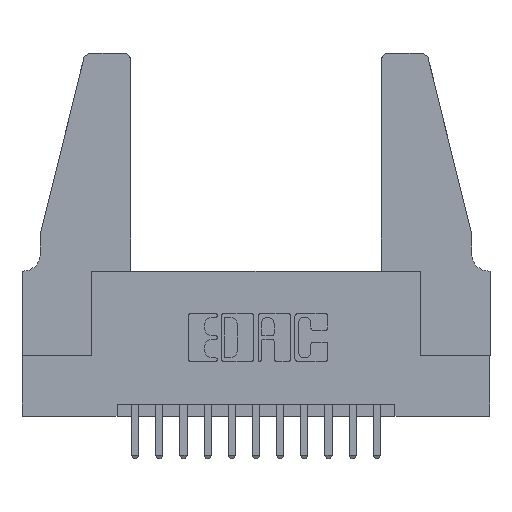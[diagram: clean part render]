
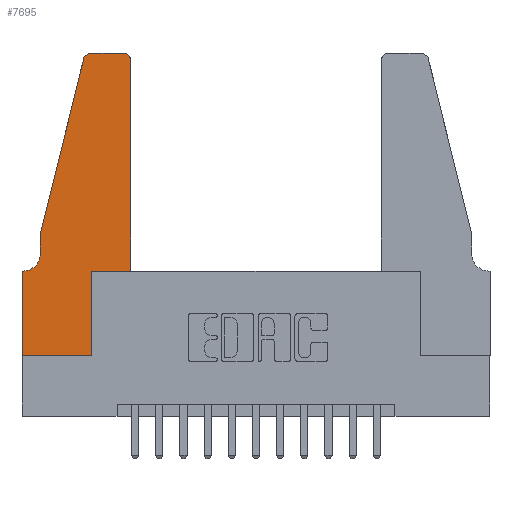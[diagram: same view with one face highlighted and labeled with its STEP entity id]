
A CAD part, top view. The second image highlights one B-rep face of the part: STEP entity #7695.
In plain terms, the highlighted planar face has unit normal (0, 0, 1).
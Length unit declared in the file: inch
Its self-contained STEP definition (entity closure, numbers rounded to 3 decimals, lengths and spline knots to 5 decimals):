
#116 = LINE ( 'NONE', #12809, #12849 ) ;
#664 = CARTESIAN_POINT ( 'NONE',  ( 0., 0., 0.37 ) ) ;
#724 = DIRECTION ( 'NONE',  ( 1., 0., 0. ) ) ;
#802 = ORIENTED_EDGE ( 'NONE', *, *, #12602, .T. ) ;
#809 = DIRECTION ( 'NONE',  ( -1., 0., 0. ) ) ;
#882 = ORIENTED_EDGE ( 'NONE', *, *, #12974, .T. ) ;
#1076 = VECTOR ( 'NONE', #12308, 39.37008 ) ;
#1190 = CARTESIAN_POINT ( 'NONE',  ( 0.0755, 0.5, 0.37 ) ) ;
#1233 = LINE ( 'NONE', #2793, #14843 ) ;
#1574 = VERTEX_POINT ( 'NONE', #13726 ) ;
#1674 = DIRECTION ( 'NONE',  ( 0., 1., 0. ) ) ;
#1694 = CARTESIAN_POINT ( 'NONE',  ( 0.284, 1.22, 0.37 ) ) ;
#1744 = VECTOR ( 'NONE', #14586, 39.37008 ) ;
#1784 = DIRECTION ( 'NONE',  ( 0., 0., 1. ) ) ;
#1960 = CIRCLE ( 'NONE', #13299, 0.03 ) ;
#2003 = CARTESIAN_POINT ( 'NONE',  ( 0.0055, 0.42, 0.37 ) ) ;
#2050 = VERTEX_POINT ( 'NONE', #6355 ) ;
#2176 = ORIENTED_EDGE ( 'NONE', *, *, #3864, .T. ) ;
#2296 = VECTOR ( 'NONE', #7128, 39.37008 ) ;
#2352 = ORIENTED_EDGE ( 'NONE', *, *, #6231, .T. ) ;
#2382 = EDGE_CURVE ( 'NONE', #13150, #2510, #10688, .T. ) ;
#2480 = LINE ( 'NONE', #664, #1744 ) ;
#2510 = VERTEX_POINT ( 'NONE', #6472 ) ;
#2565 = VERTEX_POINT ( 'NONE', #11208 ) ;
#2649 = DIRECTION ( 'NONE',  ( 1., 0., 0. ) ) ;
#2748 = ORIENTED_EDGE ( 'NONE', *, *, #12108, .T. ) ;
#2793 = CARTESIAN_POINT ( 'NONE',  ( 0.4505, 0.35, 0.37 ) ) ;
#2912 = VERTEX_POINT ( 'NONE', #5567 ) ;
#3067 = ORIENTED_EDGE ( 'NONE', *, *, #14102, .T. ) ;
#3302 = VECTOR ( 'NONE', #809, 39.37008 ) ;
#3370 = DIRECTION ( 'NONE',  ( 1., 0., 0. ) ) ;
#3554 = ORIENTED_EDGE ( 'NONE', *, *, #4898, .T. ) ;
#3655 = VERTEX_POINT ( 'NONE', #12877 ) ;
#3750 = DIRECTION ( 'NONE',  ( 0., -1., 0. ) ) ;
#3800 = DIRECTION ( 'NONE',  ( -1., 0., 0. ) ) ;
#3864 = EDGE_CURVE ( 'NONE', #2565, #5216, #13246, .T. ) ;
#3972 = ORIENTED_EDGE ( 'NONE', *, *, #5103, .T. ) ;
#4064 = DIRECTION ( 'NONE',  ( -0.239, -0.971, 0. ) ) ;
#4090 = CIRCLE ( 'NONE', #9495, 0.03 ) ;
#4207 = CARTESIAN_POINT ( 'NONE',  ( 0.0755, 0.5, 0.37 ) ) ;
#4379 = AXIS2_PLACEMENT_3D ( 'NONE', #13222, #6232, #2649 ) ;
#4698 = CARTESIAN_POINT ( 'NONE',  ( 0.4505, 1.22, 0.37 ) ) ;
#4898 = EDGE_CURVE ( 'NONE', #12331, #2050, #116, .T. ) ;
#4968 = EDGE_CURVE ( 'NONE', #2510, #8676, #1233, .T. ) ;
#5053 = ORIENTED_EDGE ( 'NONE', *, *, #13996, .T. ) ;
#5103 = EDGE_CURVE ( 'NONE', #3655, #2565, #4090, .T. ) ;
#5180 = ORIENTED_EDGE ( 'NONE', *, *, #4968, .T. ) ;
#5216 = VERTEX_POINT ( 'NONE', #1190 ) ;
#5291 = CARTESIAN_POINT ( 'NONE',  ( 0.2865, 0.35, 0.37 ) ) ;
#5370 = ORIENTED_EDGE ( 'NONE', *, *, #2382, .T. ) ;
#5567 = CARTESIAN_POINT ( 'NONE',  ( 0.0755, 0.42, 0.37 ) ) ;
#5678 = DIRECTION ( 'NONE',  ( 1., 0., 0. ) ) ;
#6006 = EDGE_LOOP ( 'NONE', ( #882, #3972, #2176, #5053, #2748, #14686, #3067, #3554, #2352, #5370, #5180, #802 ) ) ;
#6071 = DIRECTION ( 'NONE',  ( 0., 0., -1. ) ) ;
#6231 = EDGE_CURVE ( 'NONE', #2050, #13150, #12128, .T. ) ;
#6232 = DIRECTION ( 'NONE',  ( 0., 0., 1. ) ) ;
#6355 = CARTESIAN_POINT ( 'NONE',  ( 0.2865, 0., 0.37 ) ) ;
#6472 = CARTESIAN_POINT ( 'NONE',  ( 0.4505, 0.35, 0.37 ) ) ;
#6601 = CARTESIAN_POINT ( 'NONE',  ( 0.0755, 0.35, 0.37 ) ) ;
#7128 = DIRECTION ( 'NONE',  ( -1., 0., 0. ) ) ;
#7695 = ADVANCED_FACE ( 'NONE', ( #14281 ), #14189, .T. ) ;
#8307 = VECTOR ( 'NONE', #3750, 39.37008 ) ;
#8676 = VERTEX_POINT ( 'NONE', #4698 ) ;
#9053 = CIRCLE ( 'NONE', #14750, 0.07 ) ;
#9401 = CARTESIAN_POINT ( 'NONE',  ( 0.2605, 1.25, 0.37 ) ) ;
#9495 = AXIS2_PLACEMENT_3D ( 'NONE', #1694, #1784, #724 ) ;
#9509 = CARTESIAN_POINT ( 'NONE',  ( 0.0755, 0.5, 0.37 ) ) ;
#9817 = VECTOR ( 'NONE', #14290, 39.37008 ) ;
#9971 = VECTOR ( 'NONE', #4064, 39.37008 ) ;
#10067 = EDGE_CURVE ( 'NONE', #1574, #13876, #14388, .T. ) ;
#10424 = LINE ( 'NONE', #9509, #8307 ) ;
#10492 = VERTEX_POINT ( 'NONE', #12836 ) ;
#10688 = LINE ( 'NONE', #10758, #9817 ) ;
#10758 = CARTESIAN_POINT ( 'NONE',  ( 0.4505, 0.35, 0.37 ) ) ;
#11208 = CARTESIAN_POINT ( 'NONE',  ( 0.25487, 1.22718, 0.37 ) ) ;
#11640 = CARTESIAN_POINT ( 'NONE',  ( 0.4205, 1.22, 0.37 ) ) ;
#12108 = EDGE_CURVE ( 'NONE', #2912, #1574, #9053, .T. ) ;
#12128 = LINE ( 'NONE', #5291, #1076 ) ;
#12293 = LINE ( 'NONE', #9401, #2296 ) ;
#12308 = DIRECTION ( 'NONE',  ( 0., 1., 0. ) ) ;
#12331 = VERTEX_POINT ( 'NONE', #13260 ) ;
#12509 = CARTESIAN_POINT ( 'NONE',  ( 0.2865, 0.35, 0.37 ) ) ;
#12602 = EDGE_CURVE ( 'NONE', #8676, #10492, #1960, .T. ) ;
#12809 = CARTESIAN_POINT ( 'NONE',  ( 0., 0., 0.37 ) ) ;
#12836 = CARTESIAN_POINT ( 'NONE',  ( 0.4205, 1.25, 0.37 ) ) ;
#12849 = VECTOR ( 'NONE', #3370, 39.37008 ) ;
#12877 = CARTESIAN_POINT ( 'NONE',  ( 0.284, 1.25, 0.37 ) ) ;
#12974 = EDGE_CURVE ( 'NONE', #10492, #3655, #12293, .T. ) ;
#13150 = VERTEX_POINT ( 'NONE', #12509 ) ;
#13222 = CARTESIAN_POINT ( 'NONE',  ( 0., 0.35, 0.37 ) ) ;
#13246 = LINE ( 'NONE', #4207, #9971 ) ;
#13260 = CARTESIAN_POINT ( 'NONE',  ( 0., 0., 0.37 ) ) ;
#13299 = AXIS2_PLACEMENT_3D ( 'NONE', #11640, #15083, #5678 ) ;
#13726 = CARTESIAN_POINT ( 'NONE',  ( 0.0055, 0.35, 0.37 ) ) ;
#13876 = VERTEX_POINT ( 'NONE', #14078 ) ;
#13996 = EDGE_CURVE ( 'NONE', #5216, #2912, #10424, .T. ) ;
#14078 = CARTESIAN_POINT ( 'NONE',  ( 0., 0.35, 0.37 ) ) ;
#14102 = EDGE_CURVE ( 'NONE', #13876, #12331, #2480, .T. ) ;
#14189 = PLANE ( 'NONE',  #4379 ) ;
#14281 = FACE_OUTER_BOUND ( 'NONE', #6006, .T. ) ;
#14290 = DIRECTION ( 'NONE',  ( 1., 0., 0. ) ) ;
#14388 = LINE ( 'NONE', #6601, #3302 ) ;
#14586 = DIRECTION ( 'NONE',  ( 0., -1., 0. ) ) ;
#14686 = ORIENTED_EDGE ( 'NONE', *, *, #10067, .T. ) ;
#14750 = AXIS2_PLACEMENT_3D ( 'NONE', #2003, #6071, #3800 ) ;
#14843 = VECTOR ( 'NONE', #1674, 39.37008 ) ;
#15083 = DIRECTION ( 'NONE',  ( 0., 0., 1. ) ) ;
